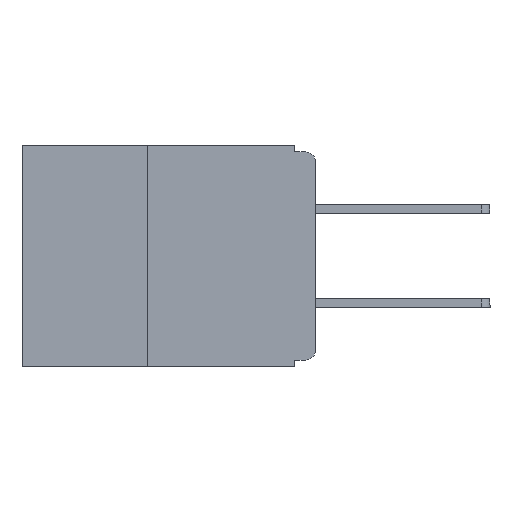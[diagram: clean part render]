
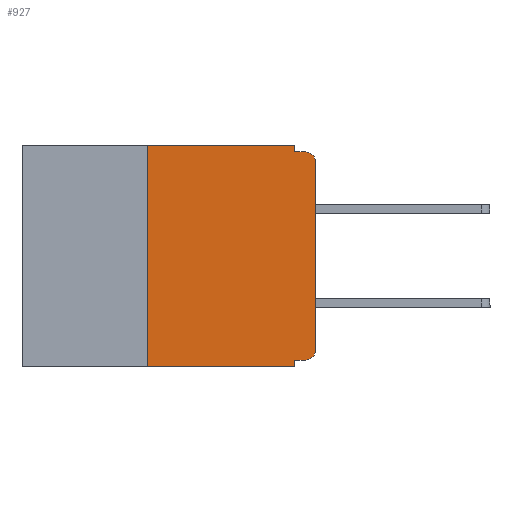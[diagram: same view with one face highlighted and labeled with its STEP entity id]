
A CAD part, left-side view. The second image highlights one B-rep face of the part: STEP entity #927.
In plain terms, the highlighted planar face has unit normal (-1, 0, 0).
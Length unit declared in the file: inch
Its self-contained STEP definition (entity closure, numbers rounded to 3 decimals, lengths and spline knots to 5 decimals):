
#47 = DIRECTION ( 'NONE',  ( 0., 1., 0. ) ) ;
#65 = LINE ( 'NONE', #1973, #4979 ) ;
#276 = CIRCLE ( 'NONE', #14029, 0.015 ) ;
#437 = FACE_OUTER_BOUND ( 'NONE', #7754, .T. ) ;
#927 = ADVANCED_FACE ( 'NONE', ( #437 ), #9574, .F. ) ;
#1081 = AXIS2_PLACEMENT_3D ( 'NONE', #17829, #17281, #16291 ) ;
#1342 = VECTOR ( 'NONE', #2350, 39.37008 ) ;
#1367 = DIRECTION ( 'NONE',  ( 0., 0., -1. ) ) ;
#1451 = CARTESIAN_POINT ( 'NONE',  ( 0., 0.031, -0.33 ) ) ;
#1949 = ORIENTED_EDGE ( 'NONE', *, *, #16771, .F. ) ;
#1951 = VECTOR ( 'NONE', #18209, 39.37008 ) ;
#1973 = CARTESIAN_POINT ( 'NONE',  ( 0., 0.437, 0. ) ) ;
#2187 = EDGE_CURVE ( 'NONE', #10113, #4212, #65, .T. ) ;
#2350 = DIRECTION ( 'NONE',  ( 0., 0., 1. ) ) ;
#2351 = CARTESIAN_POINT ( 'NONE',  ( 0., 0.031, -0.01 ) ) ;
#2835 = ORIENTED_EDGE ( 'NONE', *, *, #7236, .T. ) ;
#3532 = VERTEX_POINT ( 'NONE', #15478 ) ;
#4212 = VERTEX_POINT ( 'NONE', #21006 ) ;
#4657 = LINE ( 'NONE', #1451, #13388 ) ;
#4679 = CARTESIAN_POINT ( 'NONE',  ( 0., 0.25, 0. ) ) ;
#4743 = LINE ( 'NONE', #7915, #13983 ) ;
#4979 = VECTOR ( 'NONE', #12482, 39.37008 ) ;
#5268 = CARTESIAN_POINT ( 'NONE',  ( 0., 0., -0.01 ) ) ;
#5462 = ORIENTED_EDGE ( 'NONE', *, *, #8422, .T. ) ;
#6000 = ORIENTED_EDGE ( 'NONE', *, *, #10233, .F. ) ;
#6217 = LINE ( 'NONE', #9489, #1342 ) ;
#6230 = DIRECTION ( 'NONE',  ( 1., 0., 0. ) ) ;
#6659 = CARTESIAN_POINT ( 'NONE',  ( 0., 0.015, -0.025 ) ) ;
#6804 = LINE ( 'NONE', #8239, #1951 ) ;
#6896 = CARTESIAN_POINT ( 'NONE',  ( 0., 0.031, -0.32 ) ) ;
#7161 = CARTESIAN_POINT ( 'NONE',  ( 0., 0.437, 0. ) ) ;
#7236 = EDGE_CURVE ( 'NONE', #16718, #11337, #19591, .T. ) ;
#7581 = LINE ( 'NONE', #5268, #20259 ) ;
#7754 = EDGE_LOOP ( 'NONE', ( #9405, #11506, #14202, #14802, #15611, #19735, #5462, #6000, #1949, #2835 ) ) ;
#7909 = DIRECTION ( 'NONE',  ( 0., -1., 0. ) ) ;
#7915 = CARTESIAN_POINT ( 'NONE',  ( 0., 0.437, -0.33 ) ) ;
#8239 = CARTESIAN_POINT ( 'NONE',  ( 0., 0.25, -0.33 ) ) ;
#8422 = EDGE_CURVE ( 'NONE', #3532, #21403, #4743, .T. ) ;
#8469 = DIRECTION ( 'NONE',  ( 0., 0., -1. ) ) ;
#8498 = VERTEX_POINT ( 'NONE', #6896 ) ;
#8709 = VERTEX_POINT ( 'NONE', #2351 ) ;
#9405 = ORIENTED_EDGE ( 'NONE', *, *, #16937, .T. ) ;
#9489 = CARTESIAN_POINT ( 'NONE',  ( 0., 0., 0. ) ) ;
#9574 = PLANE ( 'NONE',  #15781 ) ;
#10012 = CARTESIAN_POINT ( 'NONE',  ( 0., 0.031, 0. ) ) ;
#10113 = VERTEX_POINT ( 'NONE', #4679 ) ;
#10233 = EDGE_CURVE ( 'NONE', #8498, #21403, #4657, .T. ) ;
#10266 = CARTESIAN_POINT ( 'NONE',  ( 0., 0.015, -0.01 ) ) ;
#10342 = LINE ( 'NONE', #10012, #19600 ) ;
#11337 = VERTEX_POINT ( 'NONE', #20408 ) ;
#11506 = ORIENTED_EDGE ( 'NONE', *, *, #18417, .T. ) ;
#12335 = DIRECTION ( 'NONE',  ( 0., 0., -1. ) ) ;
#12482 = DIRECTION ( 'NONE',  ( 0., -1., 0. ) ) ;
#12567 = CARTESIAN_POINT ( 'NONE',  ( 0., 0., -0.32 ) ) ;
#13388 = VECTOR ( 'NONE', #1367, 39.37008 ) ;
#13774 = CARTESIAN_POINT ( 'NONE',  ( 0., 0.015, -0.32 ) ) ;
#13983 = VECTOR ( 'NONE', #7909, 39.37008 ) ;
#14029 = AXIS2_PLACEMENT_3D ( 'NONE', #6659, #18425, #8469 ) ;
#14202 = ORIENTED_EDGE ( 'NONE', *, *, #21632, .F. ) ;
#14559 = LINE ( 'NONE', #12567, #18380 ) ;
#14802 = ORIENTED_EDGE ( 'NONE', *, *, #16556, .F. ) ;
#14841 = CARTESIAN_POINT ( 'NONE',  ( 0., 0., -0.025 ) ) ;
#15478 = CARTESIAN_POINT ( 'NONE',  ( 0., 0.25, -0.33 ) ) ;
#15496 = VERTEX_POINT ( 'NONE', #14841 ) ;
#15611 = ORIENTED_EDGE ( 'NONE', *, *, #2187, .F. ) ;
#15781 = AXIS2_PLACEMENT_3D ( 'NONE', #7161, #6230, #12335 ) ;
#16291 = DIRECTION ( 'NONE',  ( 0., 0., -1. ) ) ;
#16528 = EDGE_CURVE ( 'NONE', #3532, #10113, #6804, .T. ) ;
#16556 = EDGE_CURVE ( 'NONE', #4212, #8709, #10342, .T. ) ;
#16718 = VERTEX_POINT ( 'NONE', #13774 ) ;
#16771 = EDGE_CURVE ( 'NONE', #16718, #8498, #14559, .T. ) ;
#16937 = EDGE_CURVE ( 'NONE', #11337, #15496, #6217, .T. ) ;
#17281 = DIRECTION ( 'NONE',  ( -1., 0., 0. ) ) ;
#17829 = CARTESIAN_POINT ( 'NONE',  ( 0., 0.015, -0.305 ) ) ;
#18209 = DIRECTION ( 'NONE',  ( 0., 0., 1. ) ) ;
#18380 = VECTOR ( 'NONE', #47, 39.37008 ) ;
#18417 = EDGE_CURVE ( 'NONE', #15496, #20670, #276, .T. ) ;
#18425 = DIRECTION ( 'NONE',  ( -1., 0., 0. ) ) ;
#18813 = DIRECTION ( 'NONE',  ( 0., -1., 0. ) ) ;
#19591 = CIRCLE ( 'NONE', #1081, 0.015 ) ;
#19600 = VECTOR ( 'NONE', #19847, 39.37008 ) ;
#19630 = CARTESIAN_POINT ( 'NONE',  ( 0., 0.031, -0.33 ) ) ;
#19735 = ORIENTED_EDGE ( 'NONE', *, *, #16528, .F. ) ;
#19847 = DIRECTION ( 'NONE',  ( 0., 0., -1. ) ) ;
#20259 = VECTOR ( 'NONE', #18813, 39.37008 ) ;
#20408 = CARTESIAN_POINT ( 'NONE',  ( 0., 0., -0.305 ) ) ;
#20670 = VERTEX_POINT ( 'NONE', #10266 ) ;
#21006 = CARTESIAN_POINT ( 'NONE',  ( 0., 0.031, 0. ) ) ;
#21403 = VERTEX_POINT ( 'NONE', #19630 ) ;
#21632 = EDGE_CURVE ( 'NONE', #8709, #20670, #7581, .T. ) ;
